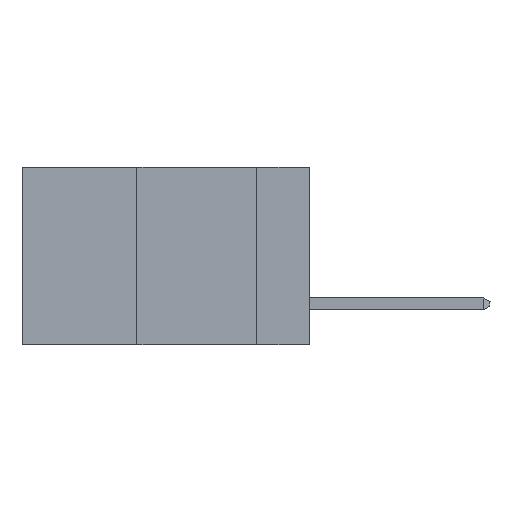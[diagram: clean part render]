
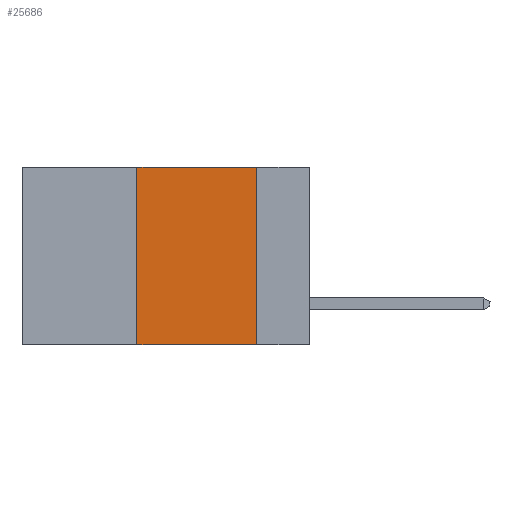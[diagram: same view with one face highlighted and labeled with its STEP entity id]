
A CAD part, left-side view. The second image highlights one B-rep face of the part: STEP entity #25686.
In plain terms, the highlighted planar face has unit normal (-1, 0, 0).
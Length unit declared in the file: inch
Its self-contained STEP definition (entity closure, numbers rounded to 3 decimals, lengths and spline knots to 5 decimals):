
#398 = CARTESIAN_POINT ( 'NONE',  ( 0., 0.11, -0.37 ) ) ;
#3011 = FACE_OUTER_BOUND ( 'NONE', #4796, .T. ) ;
#3684 = DIRECTION ( 'NONE',  ( 0., 0., 1. ) ) ;
#4796 = EDGE_LOOP ( 'NONE', ( #17603, #26642, #24105, #29741 ) ) ;
#5546 = AXIS2_PLACEMENT_3D ( 'NONE', #30158, #17493, #10378 ) ;
#5783 = CARTESIAN_POINT ( 'NONE',  ( 0., 0.36, 0. ) ) ;
#6056 = VERTEX_POINT ( 'NONE', #47247 ) ;
#8049 = VERTEX_POINT ( 'NONE', #5783 ) ;
#10378 = DIRECTION ( 'NONE',  ( 0., 0., -1. ) ) ;
#11643 = CARTESIAN_POINT ( 'NONE',  ( 0., 0.6, -0.37 ) ) ;
#12262 = DIRECTION ( 'NONE',  ( 0., 0., -1. ) ) ;
#12758 = VECTOR ( 'NONE', #12262, 39.37008 ) ;
#12962 = CARTESIAN_POINT ( 'NONE',  ( 0., 0.6, 0. ) ) ;
#17493 = DIRECTION ( 'NONE',  ( 1., 0., 0. ) ) ;
#17603 = ORIENTED_EDGE ( 'NONE', *, *, #26152, .F. ) ;
#19920 = CARTESIAN_POINT ( 'NONE',  ( 0., 0.36, 0. ) ) ;
#21972 = VECTOR ( 'NONE', #22014, 39.37008 ) ;
#21987 = VERTEX_POINT ( 'NONE', #398 ) ;
#22014 = DIRECTION ( 'NONE',  ( 0., -1., 0. ) ) ;
#22736 = LINE ( 'NONE', #19920, #48146 ) ;
#22850 = EDGE_CURVE ( 'NONE', #6056, #21987, #38779, .T. ) ;
#24105 = ORIENTED_EDGE ( 'NONE', *, *, #33376, .F. ) ;
#25686 = ADVANCED_FACE ( 'NONE', ( #3011 ), #29653, .F. ) ;
#26152 = EDGE_CURVE ( 'NONE', #47690, #21987, #40523, .T. ) ;
#26642 = ORIENTED_EDGE ( 'NONE', *, *, #42141, .F. ) ;
#29653 = PLANE ( 'NONE',  #5546 ) ;
#29741 = ORIENTED_EDGE ( 'NONE', *, *, #22850, .T. ) ;
#30158 = CARTESIAN_POINT ( 'NONE',  ( 0., 0.6, 0. ) ) ;
#33376 = EDGE_CURVE ( 'NONE', #6056, #8049, #22736, .T. ) ;
#35792 = CARTESIAN_POINT ( 'NONE',  ( 0., 0.11, 0. ) ) ;
#38779 = LINE ( 'NONE', #11643, #49863 ) ;
#39583 = LINE ( 'NONE', #12962, #21972 ) ;
#40523 = LINE ( 'NONE', #42442, #12758 ) ;
#42141 = EDGE_CURVE ( 'NONE', #8049, #47690, #39583, .T. ) ;
#42442 = CARTESIAN_POINT ( 'NONE',  ( 0., 0.11, 0. ) ) ;
#46871 = DIRECTION ( 'NONE',  ( 0., -1., 0. ) ) ;
#47247 = CARTESIAN_POINT ( 'NONE',  ( 0., 0.36, -0.37 ) ) ;
#47690 = VERTEX_POINT ( 'NONE', #35792 ) ;
#48146 = VECTOR ( 'NONE', #3684, 39.37008 ) ;
#49863 = VECTOR ( 'NONE', #46871, 39.37008 ) ;
